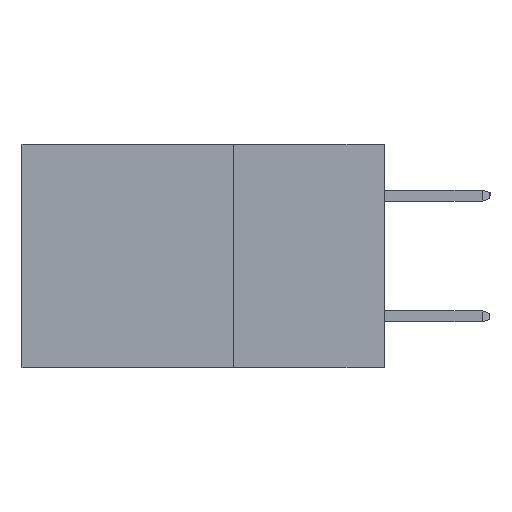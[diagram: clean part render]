
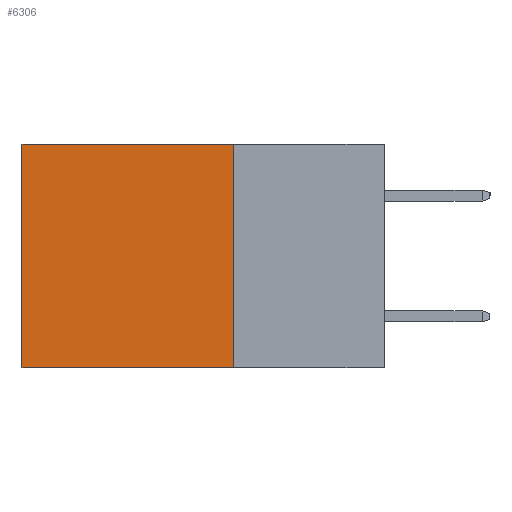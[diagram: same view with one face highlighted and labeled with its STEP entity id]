
A CAD part, left-side view. The second image highlights one B-rep face of the part: STEP entity #6306.
In plain terms, the highlighted planar face has unit normal (-1, 0, 0).
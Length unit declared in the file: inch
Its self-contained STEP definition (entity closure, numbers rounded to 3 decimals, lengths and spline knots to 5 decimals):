
#340 = CARTESIAN_POINT ( 'NONE',  ( 0.2615, 0.25, -0.37 ) ) ;
#967 = LINE ( 'NONE', #11009, #16341 ) ;
#1065 = ORIENTED_EDGE ( 'NONE', *, *, #10941, .T. ) ;
#1257 = DIRECTION ( 'NONE',  ( 1., 0., 0. ) ) ;
#2418 = CARTESIAN_POINT ( 'NONE',  ( 0.2615, 0.25, -0.37 ) ) ;
#2554 = CARTESIAN_POINT ( 'NONE',  ( 0.2615, 0.6, -0.37 ) ) ;
#2684 = CARTESIAN_POINT ( 'NONE',  ( 0.2615, 0.25, -0.37 ) ) ;
#3884 = DIRECTION ( 'NONE',  ( 0., 0., -1. ) ) ;
#4069 = CARTESIAN_POINT ( 'NONE',  ( 0.2615, 0.25, 0. ) ) ;
#4193 = VERTEX_POINT ( 'NONE', #8991 ) ;
#4817 = VERTEX_POINT ( 'NONE', #18421 ) ;
#5407 = EDGE_LOOP ( 'NONE', ( #12380, #13896, #5656, #1065 ) ) ;
#5656 = ORIENTED_EDGE ( 'NONE', *, *, #17510, .F. ) ;
#6306 = ADVANCED_FACE ( 'NONE', ( #6894 ), #11207, .F. ) ;
#6894 = FACE_OUTER_BOUND ( 'NONE', #5407, .T. ) ;
#8991 = CARTESIAN_POINT ( 'NONE',  ( 0.2615, 0.25, 0. ) ) ;
#9331 = DIRECTION ( 'NONE',  ( 0., 1., 0. ) ) ;
#9693 = VECTOR ( 'NONE', #18088, 39.37008 ) ;
#9779 = DIRECTION ( 'NONE',  ( 0., 1., 0. ) ) ;
#10095 = VERTEX_POINT ( 'NONE', #340 ) ;
#10327 = EDGE_CURVE ( 'NONE', #10095, #15866, #18070, .T. ) ;
#10941 = EDGE_CURVE ( 'NONE', #4193, #4817, #15703, .T. ) ;
#11009 = CARTESIAN_POINT ( 'NONE',  ( 0.2615, 0.6, -0.37 ) ) ;
#11207 = PLANE ( 'NONE',  #15479 ) ;
#12142 = EDGE_CURVE ( 'NONE', #4817, #15866, #967, .T. ) ;
#12380 = ORIENTED_EDGE ( 'NONE', *, *, #12142, .T. ) ;
#12700 = DIRECTION ( 'NONE',  ( 0., 0., -1. ) ) ;
#13896 = ORIENTED_EDGE ( 'NONE', *, *, #10327, .F. ) ;
#14079 = VECTOR ( 'NONE', #9779, 39.37008 ) ;
#14413 = VECTOR ( 'NONE', #9331, 39.37008 ) ;
#15001 = LINE ( 'NONE', #2418, #9693 ) ;
#15479 = AXIS2_PLACEMENT_3D ( 'NONE', #2684, #1257, #12700 ) ;
#15703 = LINE ( 'NONE', #4069, #14079 ) ;
#15866 = VERTEX_POINT ( 'NONE', #2554 ) ;
#16341 = VECTOR ( 'NONE', #3884, 39.37008 ) ;
#16381 = CARTESIAN_POINT ( 'NONE',  ( 0.2615, 0.25, -0.37 ) ) ;
#17510 = EDGE_CURVE ( 'NONE', #4193, #10095, #15001, .T. ) ;
#18070 = LINE ( 'NONE', #16381, #14413 ) ;
#18088 = DIRECTION ( 'NONE',  ( 0., 0., -1. ) ) ;
#18421 = CARTESIAN_POINT ( 'NONE',  ( 0.2615, 0.6, 0. ) ) ;
